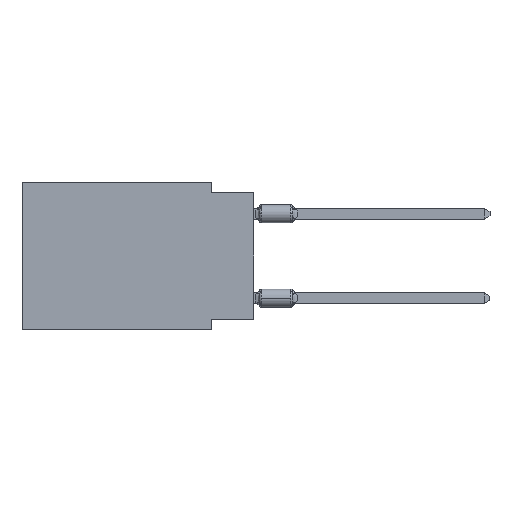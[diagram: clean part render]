
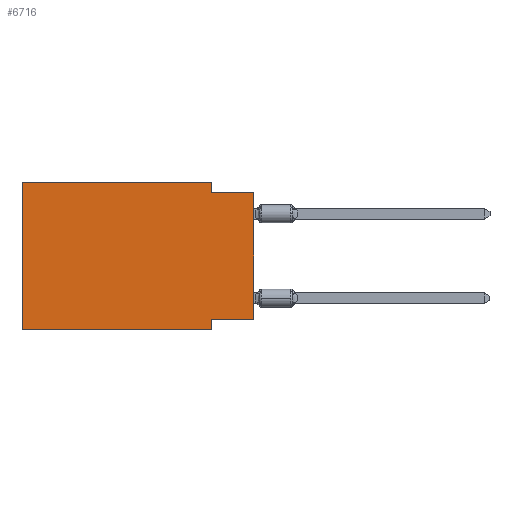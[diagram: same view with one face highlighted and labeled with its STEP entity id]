
A CAD part, left-side view. The second image highlights one B-rep face of the part: STEP entity #6716.
In plain terms, the highlighted planar face has unit normal (-1, 0, 0).
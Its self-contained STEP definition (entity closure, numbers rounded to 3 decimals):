
#192 = EDGE_CURVE ( 'NONE', #12252, #22190, #919, .T. ) ;
#576 = CARTESIAN_POINT ( 'NONE',  ( 0., 13.97, -8.89 ) ) ;
#919 = LINE ( 'NONE', #16574, #21140 ) ;
#1304 = DIRECTION ( 'NONE',  ( 0., -1., 0. ) ) ;
#1361 = DIRECTION ( 'NONE',  ( 0., 0., 1. ) ) ;
#1449 = CARTESIAN_POINT ( 'NONE',  ( 0., 13.97, 0. ) ) ;
#1512 = EDGE_LOOP ( 'NONE', ( #16381, #13825, #4054, #12067, #4808, #15827, #20270, #8392 ) ) ;
#1852 = LINE ( 'NONE', #576, #14163 ) ;
#2829 = VECTOR ( 'NONE', #1304, 1000. ) ;
#2959 = LINE ( 'NONE', #16985, #19068 ) ;
#3037 = CARTESIAN_POINT ( 'NONE',  ( 0., 13.97, 0. ) ) ;
#3119 = DIRECTION ( 'NONE',  ( 1., 0., 0. ) ) ;
#3177 = LINE ( 'NONE', #4552, #15143 ) ;
#4054 = ORIENTED_EDGE ( 'NONE', *, *, #6041, .F. ) ;
#4338 = VECTOR ( 'NONE', #1361, 1000. ) ;
#4465 = LINE ( 'NONE', #6870, #4338 ) ;
#4497 = PLANE ( 'NONE',  #9874 ) ;
#4552 = CARTESIAN_POINT ( 'NONE',  ( 0., 0., -8.255 ) ) ;
#4662 = CARTESIAN_POINT ( 'NONE',  ( 0., 0., -0.635 ) ) ;
#4719 = CARTESIAN_POINT ( 'NONE',  ( 0., 2.54, -0.635 ) ) ;
#4808 = ORIENTED_EDGE ( 'NONE', *, *, #5597, .F. ) ;
#5245 = CARTESIAN_POINT ( 'NONE',  ( 0., 0., -8.255 ) ) ;
#5597 = EDGE_CURVE ( 'NONE', #7421, #6173, #4465, .T. ) ;
#5672 = VERTEX_POINT ( 'NONE', #5245 ) ;
#6041 = EDGE_CURVE ( 'NONE', #6797, #10830, #22389, .T. ) ;
#6173 = VERTEX_POINT ( 'NONE', #1449 ) ;
#6473 = LINE ( 'NONE', #3037, #2829 ) ;
#6716 = ADVANCED_FACE ( 'NONE', ( #15444 ), #4497, .F. ) ;
#6797 = VERTEX_POINT ( 'NONE', #18541 ) ;
#6842 = DIRECTION ( 'NONE',  ( 0., 0., -1. ) ) ;
#6870 = CARTESIAN_POINT ( 'NONE',  ( 0., 13.97, 0. ) ) ;
#7195 = EDGE_CURVE ( 'NONE', #5672, #16826, #2959, .T. ) ;
#7421 = VERTEX_POINT ( 'NONE', #20052 ) ;
#8223 = DIRECTION ( 'NONE',  ( 0., -1., 0. ) ) ;
#8392 = ORIENTED_EDGE ( 'NONE', *, *, #11786, .F. ) ;
#8434 = CARTESIAN_POINT ( 'NONE',  ( 0., 2.54, -8.89 ) ) ;
#9673 = CARTESIAN_POINT ( 'NONE',  ( 0., 13.97, 0. ) ) ;
#9767 = DIRECTION ( 'NONE',  ( 0., 0., -1. ) ) ;
#9874 = AXIS2_PLACEMENT_3D ( 'NONE', #9673, #3119, #20372 ) ;
#10186 = DIRECTION ( 'NONE',  ( 0., 1., 0. ) ) ;
#10488 = EDGE_CURVE ( 'NONE', #10830, #16826, #11685, .T. ) ;
#10830 = VERTEX_POINT ( 'NONE', #4719 ) ;
#11054 = VECTOR ( 'NONE', #8223, 1000. ) ;
#11685 = LINE ( 'NONE', #4662, #11054 ) ;
#11786 = EDGE_CURVE ( 'NONE', #5672, #12252, #3177, .T. ) ;
#11803 = CARTESIAN_POINT ( 'NONE',  ( 0., 2.54, 0. ) ) ;
#12059 = VECTOR ( 'NONE', #6842, 1000. ) ;
#12067 = ORIENTED_EDGE ( 'NONE', *, *, #22079, .F. ) ;
#12252 = VERTEX_POINT ( 'NONE', #20740 ) ;
#13825 = ORIENTED_EDGE ( 'NONE', *, *, #10488, .F. ) ;
#14163 = VECTOR ( 'NONE', #19769, 1000. ) ;
#15143 = VECTOR ( 'NONE', #10186, 1000. ) ;
#15444 = FACE_OUTER_BOUND ( 'NONE', #1512, .T. ) ;
#15827 = ORIENTED_EDGE ( 'NONE', *, *, #22697, .T. ) ;
#16381 = ORIENTED_EDGE ( 'NONE', *, *, #7195, .T. ) ;
#16574 = CARTESIAN_POINT ( 'NONE',  ( 0., 2.54, -8.89 ) ) ;
#16826 = VERTEX_POINT ( 'NONE', #20444 ) ;
#16985 = CARTESIAN_POINT ( 'NONE',  ( 0., 0., 0. ) ) ;
#18541 = CARTESIAN_POINT ( 'NONE',  ( 0., 2.54, 0. ) ) ;
#18815 = DIRECTION ( 'NONE',  ( 0., 0., 1. ) ) ;
#19068 = VECTOR ( 'NONE', #18815, 1000. ) ;
#19769 = DIRECTION ( 'NONE',  ( 0., -1., 0. ) ) ;
#20052 = CARTESIAN_POINT ( 'NONE',  ( 0., 13.97, -8.89 ) ) ;
#20270 = ORIENTED_EDGE ( 'NONE', *, *, #192, .F. ) ;
#20372 = DIRECTION ( 'NONE',  ( 0., 0., -1. ) ) ;
#20444 = CARTESIAN_POINT ( 'NONE',  ( 0., 0., -0.635 ) ) ;
#20740 = CARTESIAN_POINT ( 'NONE',  ( 0., 2.54, -8.255 ) ) ;
#21140 = VECTOR ( 'NONE', #9767, 1000. ) ;
#22079 = EDGE_CURVE ( 'NONE', #6173, #6797, #6473, .T. ) ;
#22190 = VERTEX_POINT ( 'NONE', #8434 ) ;
#22389 = LINE ( 'NONE', #11803, #12059 ) ;
#22697 = EDGE_CURVE ( 'NONE', #7421, #22190, #1852, .T. ) ;
